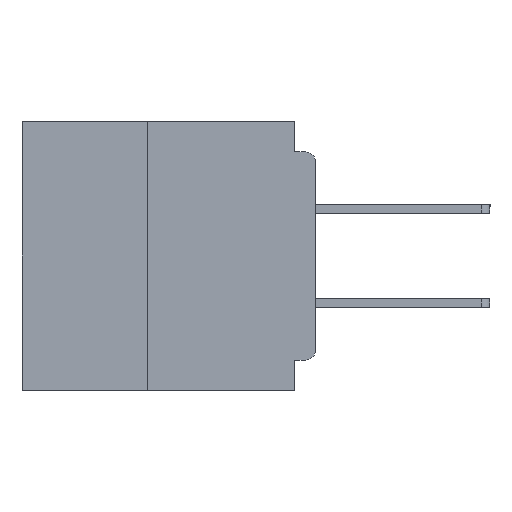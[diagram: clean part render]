
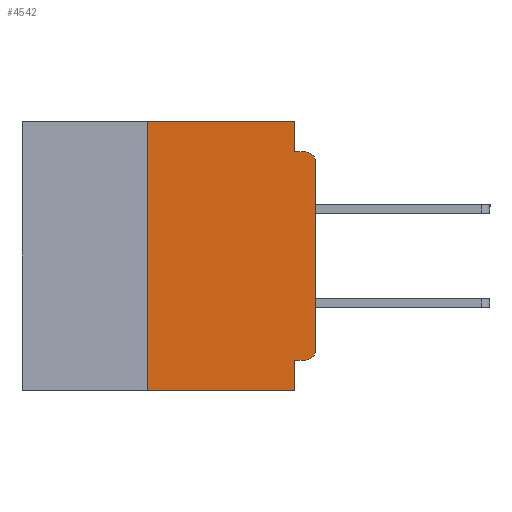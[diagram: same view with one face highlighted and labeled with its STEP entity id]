
A CAD part, left-side view. The second image highlights one B-rep face of the part: STEP entity #4542.
In plain terms, the highlighted planar face has unit normal (-1, 0, 0).
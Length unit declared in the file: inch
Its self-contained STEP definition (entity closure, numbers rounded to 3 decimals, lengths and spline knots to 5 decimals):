
#265 = EDGE_CURVE ( 'NONE', #7323, #13623, #12899, .T. ) ;
#750 = ORIENTED_EDGE ( 'NONE', *, *, #14928, .F. ) ;
#1166 = DIRECTION ( 'NONE',  ( 1., 0., 0. ) ) ;
#2074 = VECTOR ( 'NONE', #8374, 39.37008 ) ;
#2415 = VERTEX_POINT ( 'NONE', #42122 ) ;
#3012 = CARTESIAN_POINT ( 'NONE',  ( 0., 0.015, -0.355 ) ) ;
#3320 = CARTESIAN_POINT ( 'NONE',  ( 0., 0., -0.34 ) ) ;
#3591 = EDGE_CURVE ( 'NONE', #24093, #10794, #11837, .T. ) ;
#4199 = DIRECTION ( 'NONE',  ( -1., 0., 0. ) ) ;
#4306 = VERTEX_POINT ( 'NONE', #25937 ) ;
#4542 = ADVANCED_FACE ( 'NONE', ( #32668 ), #37034, .F. ) ;
#5554 = ORIENTED_EDGE ( 'NONE', *, *, #9536, .T. ) ;
#5736 = DIRECTION ( 'NONE',  ( 0., -1., 0. ) ) ;
#5798 = VERTEX_POINT ( 'NONE', #23818 ) ;
#5909 = DIRECTION ( 'NONE',  ( 0., 0., -1. ) ) ;
#6314 = ORIENTED_EDGE ( 'NONE', *, *, #35322, .F. ) ;
#6728 = ORIENTED_EDGE ( 'NONE', *, *, #31190, .F. ) ;
#7323 = VERTEX_POINT ( 'NONE', #31434 ) ;
#7909 = EDGE_LOOP ( 'NONE', ( #27164, #5554, #34598, #6728, #18697, #23301, #26022, #750, #6314, #26861 ) ) ;
#8015 = VECTOR ( 'NONE', #22956, 39.37008 ) ;
#8374 = DIRECTION ( 'NONE',  ( 0., -1., 0. ) ) ;
#8431 = DIRECTION ( 'NONE',  ( 0., 0., 1. ) ) ;
#9220 = CIRCLE ( 'NONE', #13703, 0.015 ) ;
#9369 = CARTESIAN_POINT ( 'NONE',  ( 0., 0., 0. ) ) ;
#9536 = EDGE_CURVE ( 'NONE', #13132, #10794, #9220, .T. ) ;
#9859 = CARTESIAN_POINT ( 'NONE',  ( 0., 0.031, -0.4 ) ) ;
#9966 = CARTESIAN_POINT ( 'NONE',  ( 0., 0., -0.355 ) ) ;
#10794 = VERTEX_POINT ( 'NONE', #31145 ) ;
#10795 = VECTOR ( 'NONE', #5736, 39.37008 ) ;
#11837 = LINE ( 'NONE', #25295, #10795 ) ;
#12899 = LINE ( 'NONE', #39092, #2074 ) ;
#12921 = DIRECTION ( 'NONE',  ( -1., 0., 0. ) ) ;
#13132 = VERTEX_POINT ( 'NONE', #40530 ) ;
#13623 = VERTEX_POINT ( 'NONE', #29038 ) ;
#13703 = AXIS2_PLACEMENT_3D ( 'NONE', #23824, #4199, #27083 ) ;
#14379 = VECTOR ( 'NONE', #15950, 39.37008 ) ;
#14928 = EDGE_CURVE ( 'NONE', #5798, #13623, #37381, .T. ) ;
#15753 = CARTESIAN_POINT ( 'NONE',  ( 0., 0.031, -0.045 ) ) ;
#15950 = DIRECTION ( 'NONE',  ( 0., 0., 1. ) ) ;
#16093 = EDGE_CURVE ( 'NONE', #26532, #28429, #28174, .T. ) ;
#17192 = DIRECTION ( 'NONE',  ( 0., -1., 0. ) ) ;
#18697 = ORIENTED_EDGE ( 'NONE', *, *, #31508, .F. ) ;
#19019 = VECTOR ( 'NONE', #32829, 39.37008 ) ;
#21956 = VECTOR ( 'NONE', #8431, 39.37008 ) ;
#22230 = CARTESIAN_POINT ( 'NONE',  ( 0., 0.031, 0. ) ) ;
#22956 = DIRECTION ( 'NONE',  ( 0., 1., 0. ) ) ;
#23278 = LINE ( 'NONE', #22230, #31967 ) ;
#23301 = ORIENTED_EDGE ( 'NONE', *, *, #28107, .F. ) ;
#23818 = CARTESIAN_POINT ( 'NONE',  ( 0., 0.031, -0.355 ) ) ;
#23824 = CARTESIAN_POINT ( 'NONE',  ( 0., 0.015, -0.06 ) ) ;
#24039 = DIRECTION ( 'NONE',  ( 0., 0., -1. ) ) ;
#24093 = VERTEX_POINT ( 'NONE', #15753 ) ;
#24685 = CARTESIAN_POINT ( 'NONE',  ( 0., 0.25, -0.4 ) ) ;
#25295 = CARTESIAN_POINT ( 'NONE',  ( 0., 0., -0.045 ) ) ;
#25937 = CARTESIAN_POINT ( 'NONE',  ( 0., 0.031, 0. ) ) ;
#26022 = ORIENTED_EDGE ( 'NONE', *, *, #265, .T. ) ;
#26532 = VERTEX_POINT ( 'NONE', #3012 ) ;
#26861 = ORIENTED_EDGE ( 'NONE', *, *, #16093, .T. ) ;
#27083 = DIRECTION ( 'NONE',  ( 0., 0., -1. ) ) ;
#27164 = ORIENTED_EDGE ( 'NONE', *, *, #33864, .T. ) ;
#28107 = EDGE_CURVE ( 'NONE', #7323, #2415, #41361, .T. ) ;
#28174 = CIRCLE ( 'NONE', #32765, 0.015 ) ;
#28429 = VERTEX_POINT ( 'NONE', #3320 ) ;
#29038 = CARTESIAN_POINT ( 'NONE',  ( 0., 0.031, -0.4 ) ) ;
#30663 = LINE ( 'NONE', #9369, #14379 ) ;
#31145 = CARTESIAN_POINT ( 'NONE',  ( 0., 0.015, -0.045 ) ) ;
#31190 = EDGE_CURVE ( 'NONE', #4306, #24093, #23278, .T. ) ;
#31434 = CARTESIAN_POINT ( 'NONE',  ( 0., 0.25, -0.4 ) ) ;
#31508 = EDGE_CURVE ( 'NONE', #2415, #4306, #37005, .T. ) ;
#31967 = VECTOR ( 'NONE', #5909, 39.37008 ) ;
#32448 = CARTESIAN_POINT ( 'NONE',  ( 0., 0.015, -0.34 ) ) ;
#32668 = FACE_OUTER_BOUND ( 'NONE', #7909, .T. ) ;
#32765 = AXIS2_PLACEMENT_3D ( 'NONE', #32448, #12921, #35717 ) ;
#32829 = DIRECTION ( 'NONE',  ( 0., 0., -1. ) ) ;
#33475 = CARTESIAN_POINT ( 'NONE',  ( 0., 0.437, 0. ) ) ;
#33864 = EDGE_CURVE ( 'NONE', #28429, #13132, #30663, .T. ) ;
#34051 = LINE ( 'NONE', #9966, #8015 ) ;
#34598 = ORIENTED_EDGE ( 'NONE', *, *, #3591, .F. ) ;
#35322 = EDGE_CURVE ( 'NONE', #26532, #5798, #34051, .T. ) ;
#35717 = DIRECTION ( 'NONE',  ( 0., 0., -1. ) ) ;
#35936 = AXIS2_PLACEMENT_3D ( 'NONE', #40338, #1166, #24039 ) ;
#35998 = VECTOR ( 'NONE', #17192, 39.37008 ) ;
#37005 = LINE ( 'NONE', #33475, #35998 ) ;
#37034 = PLANE ( 'NONE',  #35936 ) ;
#37381 = LINE ( 'NONE', #9859, #19019 ) ;
#39092 = CARTESIAN_POINT ( 'NONE',  ( 0., 0.437, -0.4 ) ) ;
#40338 = CARTESIAN_POINT ( 'NONE',  ( 0., 0.437, 0. ) ) ;
#40530 = CARTESIAN_POINT ( 'NONE',  ( 0., 0., -0.06 ) ) ;
#41361 = LINE ( 'NONE', #24685, #21956 ) ;
#42122 = CARTESIAN_POINT ( 'NONE',  ( 0., 0.25, 0. ) ) ;
